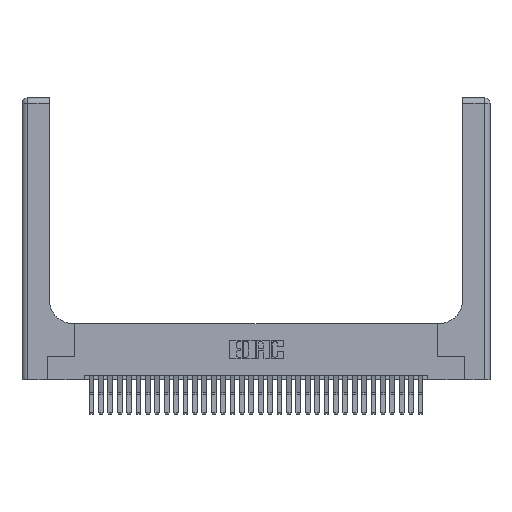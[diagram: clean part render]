
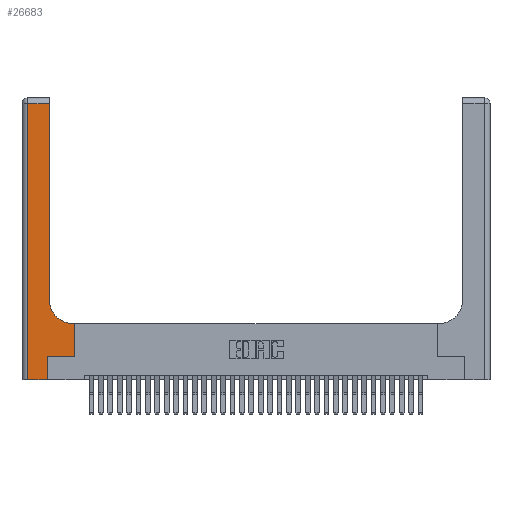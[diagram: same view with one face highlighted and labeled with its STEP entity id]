
A CAD part, top view. The second image highlights one B-rep face of the part: STEP entity #26683.
In plain terms, the highlighted planar face has unit normal (0, 0, 1).
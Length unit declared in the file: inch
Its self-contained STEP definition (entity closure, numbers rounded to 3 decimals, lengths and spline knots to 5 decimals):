
#406 = CARTESIAN_POINT ( 'NONE',  ( 0.06, 2.94, 0.37 ) ) ;
#539 = CARTESIAN_POINT ( 'NONE',  ( 0.269, 0., 0.37 ) ) ;
#1803 = EDGE_CURVE ( 'NONE', #31427, #32117, #5690, .T. ) ;
#2874 = EDGE_CURVE ( 'NONE', #16254, #11492, #9391, .T. ) ;
#2911 = ORIENTED_EDGE ( 'NONE', *, *, #17471, .T. ) ;
#2990 = EDGE_CURVE ( 'NONE', #28409, #13516, #19284, .T. ) ;
#3177 = LINE ( 'NONE', #7391, #18152 ) ;
#3203 = VECTOR ( 'NONE', #28861, 39.37008 ) ;
#3479 = ORIENTED_EDGE ( 'NONE', *, *, #34255, .T. ) ;
#3938 = DIRECTION ( 'NONE',  ( 0., 0., -1. ) ) ;
#4067 = CARTESIAN_POINT ( 'NONE',  ( 0.5415, 0.85, 0.37 ) ) ;
#4384 = ORIENTED_EDGE ( 'NONE', *, *, #21039, .T. ) ;
#4513 = CARTESIAN_POINT ( 'NONE',  ( 0.5585, 0.25, 0.37 ) ) ;
#4965 = CARTESIAN_POINT ( 'NONE',  ( 0.269, 0., 0.37 ) ) ;
#5444 = EDGE_LOOP ( 'NONE', ( #3479, #4384, #18473, #23847, #34179, #2911, #13817, #29096, #9751 ) ) ;
#5690 = LINE ( 'NONE', #4513, #8583 ) ;
#5836 = DIRECTION ( 'NONE',  ( -1., 0., 0. ) ) ;
#6909 = EDGE_CURVE ( 'NONE', #13516, #16254, #3177, .T. ) ;
#7391 = CARTESIAN_POINT ( 'NONE',  ( 0., 0., 0.37 ) ) ;
#8583 = VECTOR ( 'NONE', #25553, 39.37008 ) ;
#9391 = LINE ( 'NONE', #539, #24735 ) ;
#9751 = ORIENTED_EDGE ( 'NONE', *, *, #18816, .T. ) ;
#9795 = DIRECTION ( 'NONE',  ( 0., -1., 0. ) ) ;
#10029 = VECTOR ( 'NONE', #19125, 39.37008 ) ;
#10908 = FACE_OUTER_BOUND ( 'NONE', #5444, .T. ) ;
#10921 = DIRECTION ( 'NONE',  ( 1., 0., 0. ) ) ;
#10927 = VECTOR ( 'NONE', #5836, 39.37008 ) ;
#11492 = VERTEX_POINT ( 'NONE', #33329 ) ;
#11836 = AXIS2_PLACEMENT_3D ( 'NONE', #4067, #3938, #22523 ) ;
#12041 = VERTEX_POINT ( 'NONE', #16536 ) ;
#12235 = CARTESIAN_POINT ( 'NONE',  ( 0.06, 0., 0.37 ) ) ;
#12795 = CARTESIAN_POINT ( 'NONE',  ( 0.2915, 3., 0.37 ) ) ;
#13516 = VERTEX_POINT ( 'NONE', #12235 ) ;
#13765 = CARTESIAN_POINT ( 'NONE',  ( 0.5585, 0.25, 0.37 ) ) ;
#13791 = VERTEX_POINT ( 'NONE', #33151 ) ;
#13817 = ORIENTED_EDGE ( 'NONE', *, *, #1803, .T. ) ;
#14020 = VERTEX_POINT ( 'NONE', #32490 ) ;
#15708 = DIRECTION ( 'NONE',  ( 1., 0., 0. ) ) ;
#15748 = EDGE_CURVE ( 'NONE', #32117, #14020, #32786, .T. ) ;
#16254 = VERTEX_POINT ( 'NONE', #4965 ) ;
#16390 = VECTOR ( 'NONE', #9795, 39.37008 ) ;
#16536 = CARTESIAN_POINT ( 'NONE',  ( 0.2915, 2.94, 0.37 ) ) ;
#16870 = CARTESIAN_POINT ( 'NONE',  ( 0.5585, 0.6, 0.37 ) ) ;
#17113 = CARTESIAN_POINT ( 'NONE',  ( 0.269, 0.25, 0.37 ) ) ;
#17471 = EDGE_CURVE ( 'NONE', #11492, #31427, #33165, .T. ) ;
#18040 = LINE ( 'NONE', #29568, #10927 ) ;
#18152 = VECTOR ( 'NONE', #10921, 39.37008 ) ;
#18473 = ORIENTED_EDGE ( 'NONE', *, *, #2990, .T. ) ;
#18816 = EDGE_CURVE ( 'NONE', #14020, #13791, #27726, .T. ) ;
#19125 = DIRECTION ( 'NONE',  ( -1., 0., 0. ) ) ;
#19284 = LINE ( 'NONE', #28276, #16390 ) ;
#19736 = DIRECTION ( 'NONE',  ( -1., 0., 0. ) ) ;
#19846 = PLANE ( 'NONE',  #34180 ) ;
#21039 = EDGE_CURVE ( 'NONE', #12041, #28409, #18040, .T. ) ;
#22523 = DIRECTION ( 'NONE',  ( 1., 0., 0. ) ) ;
#23847 = ORIENTED_EDGE ( 'NONE', *, *, #6909, .T. ) ;
#24621 = DIRECTION ( 'NONE',  ( 0., 1., 0. ) ) ;
#24735 = VECTOR ( 'NONE', #24621, 39.37008 ) ;
#25553 = DIRECTION ( 'NONE',  ( 0., 1., 0. ) ) ;
#26183 = VECTOR ( 'NONE', #15708, 39.37008 ) ;
#26683 = ADVANCED_FACE ( 'NONE', ( #10908 ), #19846, .F. ) ;
#27289 = LINE ( 'NONE', #12795, #3203 ) ;
#27726 = CIRCLE ( 'NONE', #11836, 0.25 ) ;
#28276 = CARTESIAN_POINT ( 'NONE',  ( 0.06, 3., 0.37 ) ) ;
#28409 = VERTEX_POINT ( 'NONE', #406 ) ;
#28861 = DIRECTION ( 'NONE',  ( 0., 1., 0. ) ) ;
#29096 = ORIENTED_EDGE ( 'NONE', *, *, #15748, .T. ) ;
#29568 = CARTESIAN_POINT ( 'NONE',  ( 0., 2.94, 0.37 ) ) ;
#30170 = CARTESIAN_POINT ( 'NONE',  ( 0.2915, 0.6, 0.37 ) ) ;
#30441 = CARTESIAN_POINT ( 'NONE',  ( 0., 3., 0.37 ) ) ;
#31427 = VERTEX_POINT ( 'NONE', #13765 ) ;
#32117 = VERTEX_POINT ( 'NONE', #16870 ) ;
#32490 = CARTESIAN_POINT ( 'NONE',  ( 0.5415, 0.6, 0.37 ) ) ;
#32786 = LINE ( 'NONE', #30170, #10029 ) ;
#32935 = DIRECTION ( 'NONE',  ( 0., 0., -1. ) ) ;
#33151 = CARTESIAN_POINT ( 'NONE',  ( 0.2915, 0.85, 0.37 ) ) ;
#33165 = LINE ( 'NONE', #17113, #26183 ) ;
#33329 = CARTESIAN_POINT ( 'NONE',  ( 0.269, 0.25, 0.37 ) ) ;
#34179 = ORIENTED_EDGE ( 'NONE', *, *, #2874, .T. ) ;
#34180 = AXIS2_PLACEMENT_3D ( 'NONE', #30441, #32935, #19736 ) ;
#34255 = EDGE_CURVE ( 'NONE', #13791, #12041, #27289, .T. ) ;
